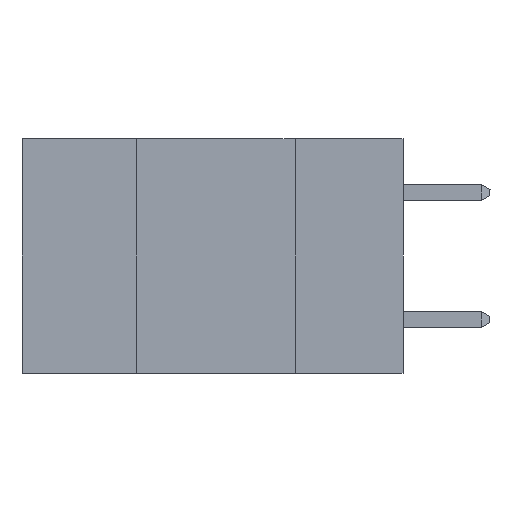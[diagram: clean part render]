
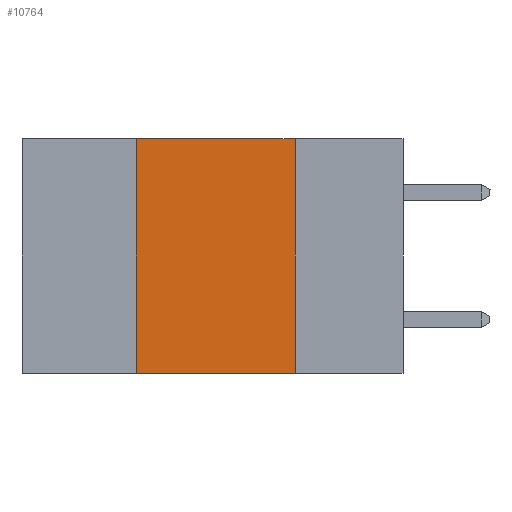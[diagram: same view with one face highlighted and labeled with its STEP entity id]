
A CAD part, left-side view. The second image highlights one B-rep face of the part: STEP entity #10764.
In plain terms, the highlighted planar face has unit normal (-1, 0, 0).
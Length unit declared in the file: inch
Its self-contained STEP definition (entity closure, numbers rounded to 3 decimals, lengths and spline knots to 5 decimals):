
#574 = DIRECTION ( 'NONE',  ( 1., 0., 0. ) ) ;
#675 = CARTESIAN_POINT ( 'NONE',  ( 0., 0.42, -0.37 ) ) ;
#1250 = VERTEX_POINT ( 'NONE', #21562 ) ;
#1282 = VECTOR ( 'NONE', #14599, 39.37008 ) ;
#2476 = VERTEX_POINT ( 'NONE', #8651 ) ;
#2704 = DIRECTION ( 'NONE',  ( 0., 0., -1. ) ) ;
#3910 = AXIS2_PLACEMENT_3D ( 'NONE', #8931, #574, #19981 ) ;
#4106 = EDGE_CURVE ( 'NONE', #2476, #8263, #6043, .T. ) ;
#4766 = CARTESIAN_POINT ( 'NONE',  ( 0., 0.17, 0. ) ) ;
#6043 = LINE ( 'NONE', #4766, #16545 ) ;
#7829 = VECTOR ( 'NONE', #16183, 39.37008 ) ;
#8263 = VERTEX_POINT ( 'NONE', #12668 ) ;
#8651 = CARTESIAN_POINT ( 'NONE',  ( 0., 0.17, 0. ) ) ;
#8931 = CARTESIAN_POINT ( 'NONE',  ( 0., 0.6, 0. ) ) ;
#9571 = ORIENTED_EDGE ( 'NONE', *, *, #18861, .T. ) ;
#10708 = LINE ( 'NONE', #12769, #21879 ) ;
#10764 = ADVANCED_FACE ( 'NONE', ( #27701 ), #21891, .F. ) ;
#12279 = VERTEX_POINT ( 'NONE', #675 ) ;
#12552 = EDGE_CURVE ( 'NONE', #1250, #2476, #15451, .T. ) ;
#12668 = CARTESIAN_POINT ( 'NONE',  ( 0., 0.17, -0.37 ) ) ;
#12769 = CARTESIAN_POINT ( 'NONE',  ( 0., 0.6, -0.37 ) ) ;
#14599 = DIRECTION ( 'NONE',  ( 0., -1., 0. ) ) ;
#14712 = ORIENTED_EDGE ( 'NONE', *, *, #21116, .F. ) ;
#14933 = DIRECTION ( 'NONE',  ( 0., -1., 0. ) ) ;
#15451 = LINE ( 'NONE', #15866, #1282 ) ;
#15866 = CARTESIAN_POINT ( 'NONE',  ( 0., 0.6, 0. ) ) ;
#16183 = DIRECTION ( 'NONE',  ( 0., 0., 1. ) ) ;
#16545 = VECTOR ( 'NONE', #2704, 39.37008 ) ;
#18438 = CARTESIAN_POINT ( 'NONE',  ( 0., 0.42, 0. ) ) ;
#18861 = EDGE_CURVE ( 'NONE', #12279, #8263, #10708, .T. ) ;
#19981 = DIRECTION ( 'NONE',  ( 0., 0., -1. ) ) ;
#20697 = LINE ( 'NONE', #18438, #7829 ) ;
#20959 = ORIENTED_EDGE ( 'NONE', *, *, #12552, .F. ) ;
#21116 = EDGE_CURVE ( 'NONE', #12279, #1250, #20697, .T. ) ;
#21562 = CARTESIAN_POINT ( 'NONE',  ( 0., 0.42, 0. ) ) ;
#21879 = VECTOR ( 'NONE', #14933, 39.37008 ) ;
#21891 = PLANE ( 'NONE',  #3910 ) ;
#26688 = ORIENTED_EDGE ( 'NONE', *, *, #4106, .F. ) ;
#27578 = EDGE_LOOP ( 'NONE', ( #26688, #20959, #14712, #9571 ) ) ;
#27701 = FACE_OUTER_BOUND ( 'NONE', #27578, .T. ) ;
